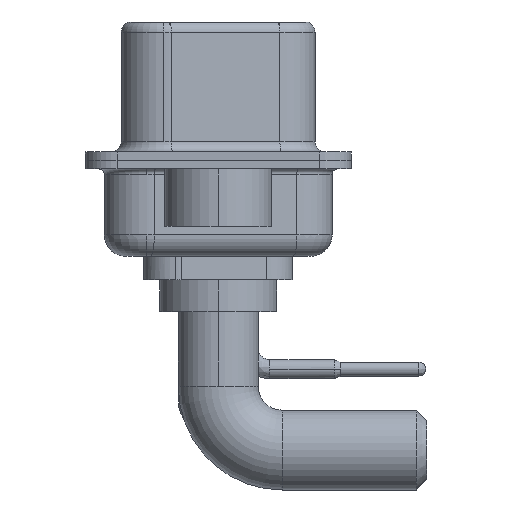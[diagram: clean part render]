
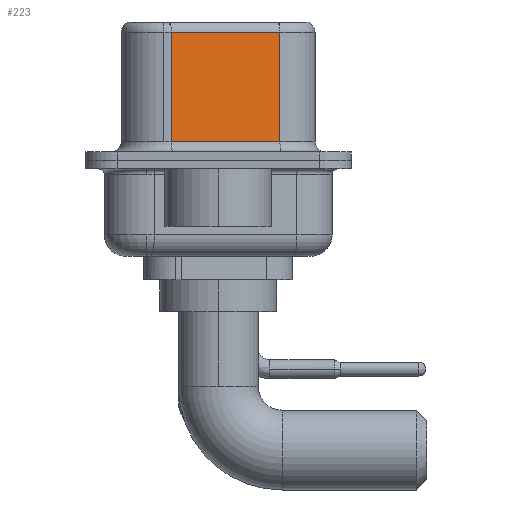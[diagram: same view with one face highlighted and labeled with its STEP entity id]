
A CAD part, left-side view. The second image highlights one B-rep face of the part: STEP entity #223.
In plain terms, the highlighted planar face has unit normal (-0.985, -0.174, 0).
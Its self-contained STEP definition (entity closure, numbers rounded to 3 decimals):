
#223 = ADVANCED_FACE ( 'NONE', ( #17194 ), #25479, .F. ) ;
#2711 = ORIENTED_EDGE ( 'NONE', *, *, #10437, .T. ) ;
#3462 = DIRECTION ( 'NONE',  ( 0., 0., -1. ) ) ;
#4360 = VERTEX_POINT ( 'NONE', #25189 ) ;
#4604 = CARTESIAN_POINT ( 'NONE',  ( 4.58, -2.897, 6.02 ) ) ;
#5630 = LINE ( 'NONE', #25836, #21812 ) ;
#6437 = ORIENTED_EDGE ( 'NONE', *, *, #23120, .F. ) ;
#6697 = LINE ( 'NONE', #12677, #15568 ) ;
#6893 = CARTESIAN_POINT ( 'NONE',  ( 4.58, -2.897, 6.52 ) ) ;
#8570 = VECTOR ( 'NONE', #15414, 1000. ) ;
#9131 = CARTESIAN_POINT ( 'NONE',  ( 3.68, 2.203, 0.9 ) ) ;
#9197 = CARTESIAN_POINT ( 'NONE',  ( 4.58, -2.897, 0.9 ) ) ;
#10437 = EDGE_CURVE ( 'NONE', #15839, #24062, #19369, .T. ) ;
#12161 = EDGE_CURVE ( 'NONE', #14257, #4360, #6697, .T. ) ;
#12677 = CARTESIAN_POINT ( 'NONE',  ( 4.58, -2.897, 6.02 ) ) ;
#12993 = DIRECTION ( 'NONE',  ( 0.985, 0.174, 0. ) ) ;
#13033 = DIRECTION ( 'NONE',  ( 0., 0., -1. ) ) ;
#13449 = ORIENTED_EDGE ( 'NONE', *, *, #14451, .T. ) ;
#14257 = VERTEX_POINT ( 'NONE', #4604 ) ;
#14451 = EDGE_CURVE ( 'NONE', #4360, #15839, #5630, .T. ) ;
#15414 = DIRECTION ( 'NONE',  ( 0.174, -0.985, 0. ) ) ;
#15568 = VECTOR ( 'NONE', #20960, 1000. ) ;
#15839 = VERTEX_POINT ( 'NONE', #9131 ) ;
#16970 = LINE ( 'NONE', #18875, #18534 ) ;
#17194 = FACE_OUTER_BOUND ( 'NONE', #22106, .T. ) ;
#17645 = AXIS2_PLACEMENT_3D ( 'NONE', #6893, #12993, #21279 ) ;
#18534 = VECTOR ( 'NONE', #13033, 1000. ) ;
#18875 = CARTESIAN_POINT ( 'NONE',  ( 4.58, -2.897, 6.52 ) ) ;
#19369 = LINE ( 'NONE', #23564, #8570 ) ;
#20960 = DIRECTION ( 'NONE',  ( -0.174, 0.985, 0. ) ) ;
#21279 = DIRECTION ( 'NONE',  ( -0.174, 0.985, 0. ) ) ;
#21812 = VECTOR ( 'NONE', #3462, 1000. ) ;
#22106 = EDGE_LOOP ( 'NONE', ( #6437, #25474, #13449, #2711 ) ) ;
#23120 = EDGE_CURVE ( 'NONE', #14257, #24062, #16970, .T. ) ;
#23564 = CARTESIAN_POINT ( 'NONE',  ( 4.58, -2.897, 0.9 ) ) ;
#24062 = VERTEX_POINT ( 'NONE', #9197 ) ;
#25189 = CARTESIAN_POINT ( 'NONE',  ( 3.68, 2.203, 6.02 ) ) ;
#25474 = ORIENTED_EDGE ( 'NONE', *, *, #12161, .T. ) ;
#25479 = PLANE ( 'NONE',  #17645 ) ;
#25836 = CARTESIAN_POINT ( 'NONE',  ( 3.68, 2.203, 6.52 ) ) ;
